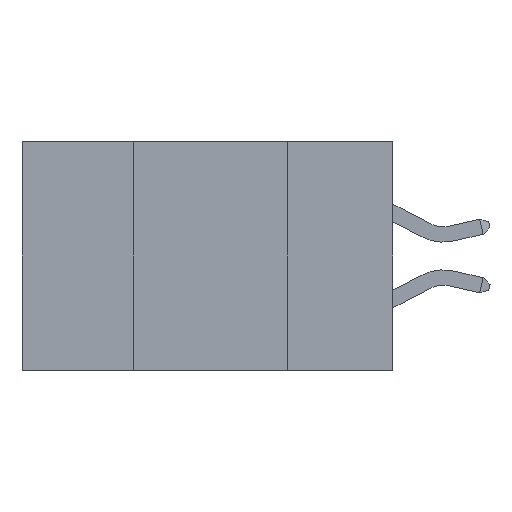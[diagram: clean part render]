
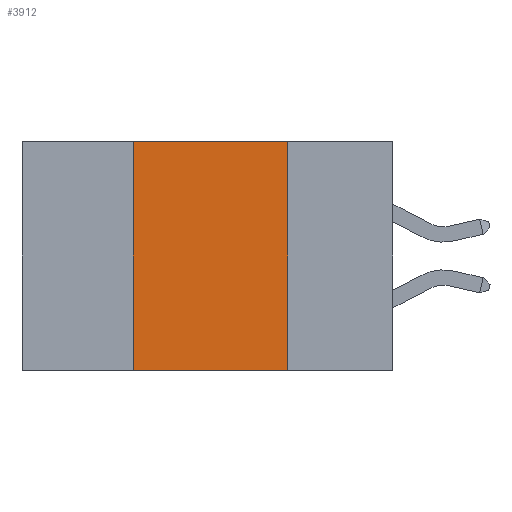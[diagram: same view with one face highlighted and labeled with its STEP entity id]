
A CAD part, left-side view. The second image highlights one B-rep face of the part: STEP entity #3912.
In plain terms, the highlighted planar face has unit normal (-1, 0, 0).
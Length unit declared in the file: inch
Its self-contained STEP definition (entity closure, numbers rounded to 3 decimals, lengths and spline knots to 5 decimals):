
#94 = DIRECTION ( 'NONE',  ( 0., 0., -1. ) ) ;
#345 = DIRECTION ( 'NONE',  ( 0., 0., 1. ) ) ;
#1281 = CARTESIAN_POINT ( 'NONE',  ( 0., 0.6, 0. ) ) ;
#1797 = VERTEX_POINT ( 'NONE', #3990 ) ;
#2686 = EDGE_CURVE ( 'NONE', #4381, #17240, #17463, .T. ) ;
#3156 = CARTESIAN_POINT ( 'NONE',  ( 0., 0.6, -0.37 ) ) ;
#3249 = CARTESIAN_POINT ( 'NONE',  ( 0., 0.42, -0.37 ) ) ;
#3647 = EDGE_LOOP ( 'NONE', ( #8630, #7629, #17323, #15100 ) ) ;
#3912 = ADVANCED_FACE ( 'NONE', ( #10876 ), #17304, .F. ) ;
#3990 = CARTESIAN_POINT ( 'NONE',  ( 0., 0.17, -0.37 ) ) ;
#4381 = VERTEX_POINT ( 'NONE', #17312 ) ;
#5044 = VERTEX_POINT ( 'NONE', #3249 ) ;
#6054 = CARTESIAN_POINT ( 'NONE',  ( 0., 0.17, 0. ) ) ;
#6243 = CARTESIAN_POINT ( 'NONE',  ( 0., 0.42, 0. ) ) ;
#6259 = LINE ( 'NONE', #10215, #16337 ) ;
#6355 = VECTOR ( 'NONE', #11714, 39.37008 ) ;
#7048 = LINE ( 'NONE', #3156, #6355 ) ;
#7146 = VECTOR ( 'NONE', #14524, 39.37008 ) ;
#7552 = AXIS2_PLACEMENT_3D ( 'NONE', #8497, #8572, #11901 ) ;
#7629 = ORIENTED_EDGE ( 'NONE', *, *, #2686, .F. ) ;
#7999 = LINE ( 'NONE', #6243, #13774 ) ;
#8497 = CARTESIAN_POINT ( 'NONE',  ( 0., 0.6, 0. ) ) ;
#8572 = DIRECTION ( 'NONE',  ( 1., 0., 0. ) ) ;
#8630 = ORIENTED_EDGE ( 'NONE', *, *, #9903, .F. ) ;
#9903 = EDGE_CURVE ( 'NONE', #17240, #1797, #6259, .T. ) ;
#10215 = CARTESIAN_POINT ( 'NONE',  ( 0., 0.17, 0. ) ) ;
#10876 = FACE_OUTER_BOUND ( 'NONE', #3647, .T. ) ;
#11714 = DIRECTION ( 'NONE',  ( 0., -1., 0. ) ) ;
#11901 = DIRECTION ( 'NONE',  ( 0., 0., -1. ) ) ;
#13774 = VECTOR ( 'NONE', #345, 39.37008 ) ;
#14524 = DIRECTION ( 'NONE',  ( 0., -1., 0. ) ) ;
#15100 = ORIENTED_EDGE ( 'NONE', *, *, #18750, .T. ) ;
#16337 = VECTOR ( 'NONE', #94, 39.37008 ) ;
#17240 = VERTEX_POINT ( 'NONE', #6054 ) ;
#17304 = PLANE ( 'NONE',  #7552 ) ;
#17312 = CARTESIAN_POINT ( 'NONE',  ( 0., 0.42, 0. ) ) ;
#17323 = ORIENTED_EDGE ( 'NONE', *, *, #17413, .F. ) ;
#17413 = EDGE_CURVE ( 'NONE', #5044, #4381, #7999, .T. ) ;
#17463 = LINE ( 'NONE', #1281, #7146 ) ;
#18750 = EDGE_CURVE ( 'NONE', #5044, #1797, #7048, .T. ) ;
